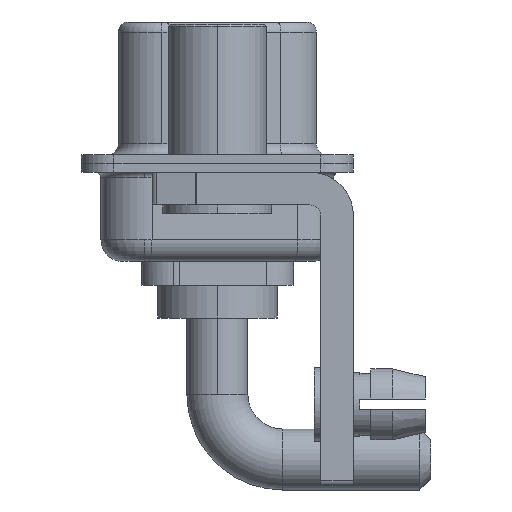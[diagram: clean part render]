
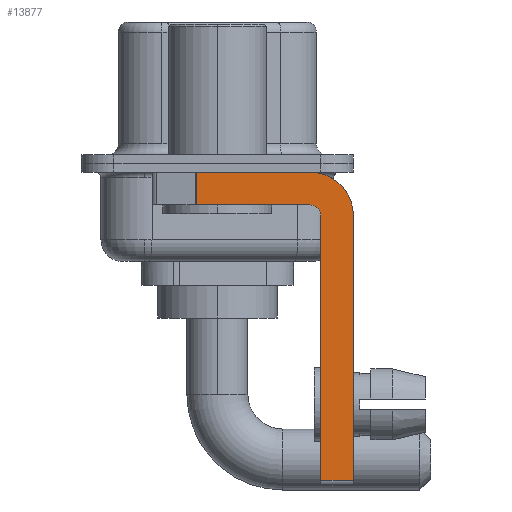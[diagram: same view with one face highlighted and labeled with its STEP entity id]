
A CAD part, left-side view. The second image highlights one B-rep face of the part: STEP entity #13877.
In plain terms, the highlighted planar face has unit normal (-1, 0, 0).
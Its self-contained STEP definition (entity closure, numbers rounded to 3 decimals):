
#394 = CARTESIAN_POINT ( 'NONE',  ( -2.9, -6.25, -2.4 ) ) ;
#407 = DIRECTION ( 'NONE',  ( 0., 0., -1. ) ) ;
#423 = DIRECTION ( 'NONE',  ( 0., 1., 0. ) ) ;
#738 = VECTOR ( 'NONE', #15185, 1000. ) ;
#811 = ORIENTED_EDGE ( 'NONE', *, *, #11079, .F. ) ;
#1123 = CARTESIAN_POINT ( 'NONE',  ( -2.9, -4.25, -14.55 ) ) ;
#1869 = AXIS2_PLACEMENT_3D ( 'NONE', #3190, #8739, #13141 ) ;
#1998 = CARTESIAN_POINT ( 'NONE',  ( -2.9, -4.25, -1.9 ) ) ;
#2187 = EDGE_CURVE ( 'NONE', #11172, #11235, #9965, .T. ) ;
#3153 = VECTOR ( 'NONE', #13753, 1000. ) ;
#3190 = CARTESIAN_POINT ( 'NONE',  ( -2.9, -4.25, -2.4 ) ) ;
#3875 = CARTESIAN_POINT ( 'NONE',  ( -2.9, -4.75, -2.4 ) ) ;
#4077 = VECTOR ( 'NONE', #13912, 1000. ) ;
#4508 = PLANE ( 'NONE',  #5058 ) ;
#4656 = VECTOR ( 'NONE', #15159, 1000. ) ;
#4922 = CARTESIAN_POINT ( 'NONE',  ( -2.9, -4.75, -14.8 ) ) ;
#5058 = AXIS2_PLACEMENT_3D ( 'NONE', #11927, #10152, #407 ) ;
#5199 = LINE ( 'NONE', #4922, #3153 ) ;
#5275 = VERTEX_POINT ( 'NONE', #394 ) ;
#5562 = AXIS2_PLACEMENT_3D ( 'NONE', #12236, #16093, #8970 ) ;
#5607 = EDGE_CURVE ( 'NONE', #14290, #6276, #18358, .T. ) ;
#5671 = CARTESIAN_POINT ( 'NONE',  ( -2.9, -6.25, -14.55 ) ) ;
#5736 = EDGE_LOOP ( 'NONE', ( #811, #8938, #8697, #7127, #15725, #9088, #11003, #16001 ) ) ;
#6276 = VERTEX_POINT ( 'NONE', #5671 ) ;
#6704 = VERTEX_POINT ( 'NONE', #14487 ) ;
#6861 = EDGE_CURVE ( 'NONE', #11235, #8845, #14580, .T. ) ;
#7127 = ORIENTED_EDGE ( 'NONE', *, *, #2187, .F. ) ;
#7853 = EDGE_CURVE ( 'NONE', #6704, #5275, #12471, .T. ) ;
#8170 = CARTESIAN_POINT ( 'NONE',  ( -2.9, 0.978, -0.4 ) ) ;
#8358 = EDGE_CURVE ( 'NONE', #14310, #8845, #10993, .T. ) ;
#8660 = FACE_OUTER_BOUND ( 'NONE', #5736, .T. ) ;
#8697 = ORIENTED_EDGE ( 'NONE', *, *, #6861, .F. ) ;
#8739 = DIRECTION ( 'NONE',  ( -1., 0., 0. ) ) ;
#8845 = VERTEX_POINT ( 'NONE', #10784 ) ;
#8938 = ORIENTED_EDGE ( 'NONE', *, *, #8358, .T. ) ;
#8970 = DIRECTION ( 'NONE',  ( 0., 0., -1. ) ) ;
#9088 = ORIENTED_EDGE ( 'NONE', *, *, #5607, .T. ) ;
#9429 = CARTESIAN_POINT ( 'NONE',  ( -2.9, 3., -0.4 ) ) ;
#9738 = VECTOR ( 'NONE', #423, 1000. ) ;
#9833 = DIRECTION ( 'NONE',  ( 0., -1., 0. ) ) ;
#9942 = CARTESIAN_POINT ( 'NONE',  ( -2.9, -4.75, -14.55 ) ) ;
#9965 = CIRCLE ( 'NONE', #1869, 0.5 ) ;
#10152 = DIRECTION ( 'NONE',  ( 1., 0., 0. ) ) ;
#10485 = EDGE_CURVE ( 'NONE', #5275, #6276, #17981, .T. ) ;
#10784 = CARTESIAN_POINT ( 'NONE',  ( -2.9, 0.978, -1.9 ) ) ;
#10993 = LINE ( 'NONE', #11178, #4077 ) ;
#11003 = ORIENTED_EDGE ( 'NONE', *, *, #10485, .F. ) ;
#11005 = EDGE_CURVE ( 'NONE', #14290, #11172, #5199, .T. ) ;
#11079 = EDGE_CURVE ( 'NONE', #14310, #6704, #16562, .T. ) ;
#11172 = VERTEX_POINT ( 'NONE', #3875 ) ;
#11178 = CARTESIAN_POINT ( 'NONE',  ( -2.9, 0.978, -1.9 ) ) ;
#11235 = VERTEX_POINT ( 'NONE', #14300 ) ;
#11927 = CARTESIAN_POINT ( 'NONE',  ( -2.9, -4.25, -2.4 ) ) ;
#12236 = CARTESIAN_POINT ( 'NONE',  ( -2.9, -4.25, -2.4 ) ) ;
#12471 = CIRCLE ( 'NONE', #5562, 2. ) ;
#13141 = DIRECTION ( 'NONE',  ( 0., 0., 1. ) ) ;
#13753 = DIRECTION ( 'NONE',  ( 0., 0., 1. ) ) ;
#13877 = ADVANCED_FACE ( 'NONE', ( #8660 ), #4508, .F. ) ;
#13912 = DIRECTION ( 'NONE',  ( 0., 0., -1. ) ) ;
#14290 = VERTEX_POINT ( 'NONE', #9942 ) ;
#14300 = CARTESIAN_POINT ( 'NONE',  ( -2.9, -4.25, -1.9 ) ) ;
#14310 = VERTEX_POINT ( 'NONE', #8170 ) ;
#14487 = CARTESIAN_POINT ( 'NONE',  ( -2.9, -4.25, -0.4 ) ) ;
#14580 = LINE ( 'NONE', #1998, #9738 ) ;
#15159 = DIRECTION ( 'NONE',  ( 0., -1., 0. ) ) ;
#15185 = DIRECTION ( 'NONE',  ( 0., 0., -1. ) ) ;
#15271 = CARTESIAN_POINT ( 'NONE',  ( -2.9, -6.25, -2.4 ) ) ;
#15725 = ORIENTED_EDGE ( 'NONE', *, *, #11005, .F. ) ;
#16001 = ORIENTED_EDGE ( 'NONE', *, *, #7853, .F. ) ;
#16039 = VECTOR ( 'NONE', #9833, 1000. ) ;
#16093 = DIRECTION ( 'NONE',  ( 1., 0., 0. ) ) ;
#16562 = LINE ( 'NONE', #9429, #4656 ) ;
#17981 = LINE ( 'NONE', #15271, #738 ) ;
#18358 = LINE ( 'NONE', #1123, #16039 ) ;
